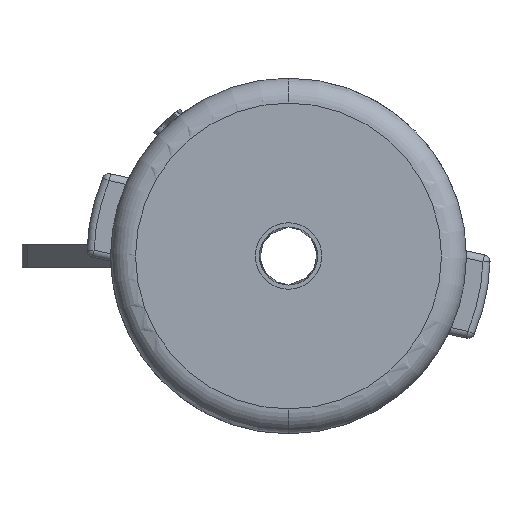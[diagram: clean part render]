
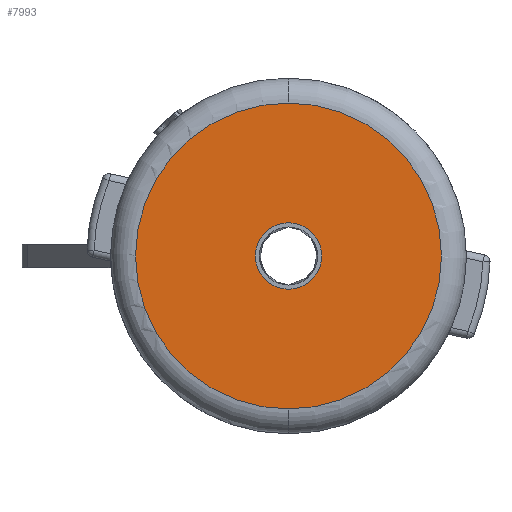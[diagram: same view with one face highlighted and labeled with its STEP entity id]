
A CAD part, front view. The second image highlights one B-rep face of the part: STEP entity #7993.
In plain terms, the highlighted planar face has unit normal (0, -1, 0).
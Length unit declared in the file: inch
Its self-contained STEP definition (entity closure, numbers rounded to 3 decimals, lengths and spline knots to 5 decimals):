
#191 = EDGE_LOOP ( 'NONE', ( #3688, #3176 ) ) ;
#700 = VERTEX_POINT ( 'NONE', #10809 ) ;
#851 = VERTEX_POINT ( 'NONE', #2361 ) ;
#1659 = AXIS2_PLACEMENT_3D ( 'NONE', #2251, #8690, #3186 ) ;
#1875 = DIRECTION ( 'NONE',  ( 0., -1., 0. ) ) ;
#2243 = CIRCLE ( 'NONE', #6892, 0.14 ) ;
#2251 = CARTESIAN_POINT ( 'NONE',  ( 0., 0., 0. ) ) ;
#2307 = DIRECTION ( 'NONE',  ( 0., 0., -1. ) ) ;
#2361 = CARTESIAN_POINT ( 'NONE',  ( 0., 0., 0.14 ) ) ;
#2956 = EDGE_LOOP ( 'NONE', ( #4326, #8024 ) ) ;
#2997 = CARTESIAN_POINT ( 'NONE',  ( 0., 0., 0. ) ) ;
#3078 = EDGE_CURVE ( 'NONE', #851, #8183, #2243, .T. ) ;
#3131 = AXIS2_PLACEMENT_3D ( 'NONE', #4137, #7835, #2307 ) ;
#3176 = ORIENTED_EDGE ( 'NONE', *, *, #3078, .T. ) ;
#3186 = DIRECTION ( 'NONE',  ( 0., 0., 1. ) ) ;
#3676 = CARTESIAN_POINT ( 'NONE',  ( 0., 0., 0. ) ) ;
#3688 = ORIENTED_EDGE ( 'NONE', *, *, #8498, .T. ) ;
#3933 = DIRECTION ( 'NONE',  ( 0., 0., 1. ) ) ;
#4137 = CARTESIAN_POINT ( 'NONE',  ( 0., 0., 0. ) ) ;
#4326 = ORIENTED_EDGE ( 'NONE', *, *, #10136, .T. ) ;
#4612 = DIRECTION ( 'NONE',  ( 0., 0., -1. ) ) ;
#5125 = CIRCLE ( 'NONE', #8286, 0.645 ) ;
#6892 = AXIS2_PLACEMENT_3D ( 'NONE', #2997, #9439, #3933 ) ;
#6904 = PLANE ( 'NONE',  #3131 ) ;
#6980 = FACE_OUTER_BOUND ( 'NONE', #2956, .T. ) ;
#7266 = FACE_BOUND ( 'NONE', #191, .T. ) ;
#7399 = CARTESIAN_POINT ( 'NONE',  ( 0., 0., 0. ) ) ;
#7688 = CIRCLE ( 'NONE', #1659, 0.14 ) ;
#7835 = DIRECTION ( 'NONE',  ( 0., -1., 0. ) ) ;
#7892 = CARTESIAN_POINT ( 'NONE',  ( 0., 0., 0.645 ) ) ;
#7941 = EDGE_CURVE ( 'NONE', #10546, #700, #5125, .T. ) ;
#7993 = ADVANCED_FACE ( 'NONE', ( #6980, #7266 ), #6904, .T. ) ;
#8024 = ORIENTED_EDGE ( 'NONE', *, *, #7941, .T. ) ;
#8183 = VERTEX_POINT ( 'NONE', #8295 ) ;
#8286 = AXIS2_PLACEMENT_3D ( 'NONE', #3676, #10129, #4612 ) ;
#8295 = CARTESIAN_POINT ( 'NONE',  ( 0., 0., -0.14 ) ) ;
#8318 = DIRECTION ( 'NONE',  ( 0., 0., -1. ) ) ;
#8498 = EDGE_CURVE ( 'NONE', #8183, #851, #7688, .T. ) ;
#8520 = AXIS2_PLACEMENT_3D ( 'NONE', #7399, #1875, #8318 ) ;
#8690 = DIRECTION ( 'NONE',  ( 0., 1., 0. ) ) ;
#9439 = DIRECTION ( 'NONE',  ( 0., 1., 0. ) ) ;
#10129 = DIRECTION ( 'NONE',  ( 0., -1., 0. ) ) ;
#10136 = EDGE_CURVE ( 'NONE', #700, #10546, #10140, .T. ) ;
#10140 = CIRCLE ( 'NONE', #8520, 0.645 ) ;
#10546 = VERTEX_POINT ( 'NONE', #7892 ) ;
#10809 = CARTESIAN_POINT ( 'NONE',  ( 0., 0., -0.645 ) ) ;
